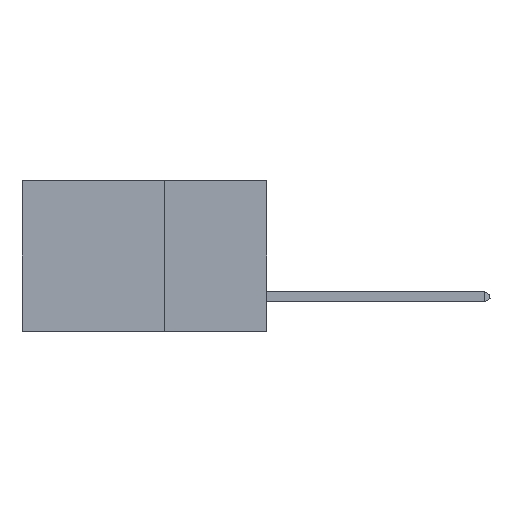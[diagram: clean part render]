
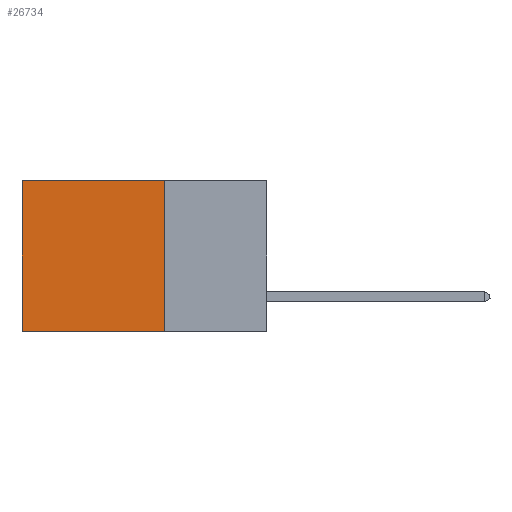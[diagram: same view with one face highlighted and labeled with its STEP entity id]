
A CAD part, left-side view. The second image highlights one B-rep face of the part: STEP entity #26734.
In plain terms, the highlighted planar face has unit normal (-1, 0, 0).
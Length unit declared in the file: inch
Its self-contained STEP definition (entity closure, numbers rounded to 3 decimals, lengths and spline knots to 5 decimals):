
#4396 = LINE ( 'NONE', #17315, #47595 ) ;
#5130 = CARTESIAN_POINT ( 'NONE',  ( 0.2875, 0.6, 0. ) ) ;
#6138 = LINE ( 'NONE', #26392, #39903 ) ;
#7076 = AXIS2_PLACEMENT_3D ( 'NONE', #45685, #40576, #45865 ) ;
#9690 = PLANE ( 'NONE',  #7076 ) ;
#11486 = CARTESIAN_POINT ( 'NONE',  ( 0.2875, 0.25, 0. ) ) ;
#12282 = EDGE_CURVE ( 'NONE', #30151, #20184, #4396, .T. ) ;
#12560 = EDGE_CURVE ( 'NONE', #30151, #24450, #6138, .T. ) ;
#17315 = CARTESIAN_POINT ( 'NONE',  ( 0.2875, 0.25, 0. ) ) ;
#17717 = ORIENTED_EDGE ( 'NONE', *, *, #34942, .T. ) ;
#18763 = ORIENTED_EDGE ( 'NONE', *, *, #12560, .F. ) ;
#19027 = EDGE_LOOP ( 'NONE', ( #17717, #40004, #18763, #41364 ) ) ;
#20184 = VERTEX_POINT ( 'NONE', #27839 ) ;
#20210 = DIRECTION ( 'NONE',  ( 0., 0., -1. ) ) ;
#24450 = VERTEX_POINT ( 'NONE', #28036 ) ;
#25936 = CARTESIAN_POINT ( 'NONE',  ( 0.2875, 0.6, -0.37 ) ) ;
#26392 = CARTESIAN_POINT ( 'NONE',  ( 0.2875, 0.25, 0. ) ) ;
#26556 = DIRECTION ( 'NONE',  ( 0., 0., -1. ) ) ;
#26720 = VECTOR ( 'NONE', #20210, 39.37008 ) ;
#26734 = ADVANCED_FACE ( 'NONE', ( #39041 ), #9690, .F. ) ;
#27839 = CARTESIAN_POINT ( 'NONE',  ( 0.2875, 0.6, 0. ) ) ;
#28036 = CARTESIAN_POINT ( 'NONE',  ( 0.2875, 0.25, -0.37 ) ) ;
#30098 = VECTOR ( 'NONE', #48770, 39.37008 ) ;
#30151 = VERTEX_POINT ( 'NONE', #11486 ) ;
#32846 = EDGE_CURVE ( 'NONE', #24450, #46514, #40179, .T. ) ;
#34942 = EDGE_CURVE ( 'NONE', #20184, #46514, #35586, .T. ) ;
#35586 = LINE ( 'NONE', #5130, #26720 ) ;
#39041 = FACE_OUTER_BOUND ( 'NONE', #19027, .T. ) ;
#39903 = VECTOR ( 'NONE', #26556, 39.37008 ) ;
#40004 = ORIENTED_EDGE ( 'NONE', *, *, #32846, .F. ) ;
#40179 = LINE ( 'NONE', #41874, #30098 ) ;
#40576 = DIRECTION ( 'NONE',  ( 1., 0., 0. ) ) ;
#41364 = ORIENTED_EDGE ( 'NONE', *, *, #12282, .T. ) ;
#41874 = CARTESIAN_POINT ( 'NONE',  ( 0.2875, 0.25, -0.37 ) ) ;
#43767 = DIRECTION ( 'NONE',  ( 0., 1., 0. ) ) ;
#45685 = CARTESIAN_POINT ( 'NONE',  ( 0.2875, 0.25, 0. ) ) ;
#45865 = DIRECTION ( 'NONE',  ( 0., 0., -1. ) ) ;
#46514 = VERTEX_POINT ( 'NONE', #25936 ) ;
#47595 = VECTOR ( 'NONE', #43767, 39.37008 ) ;
#48770 = DIRECTION ( 'NONE',  ( 0., 1., 0. ) ) ;
